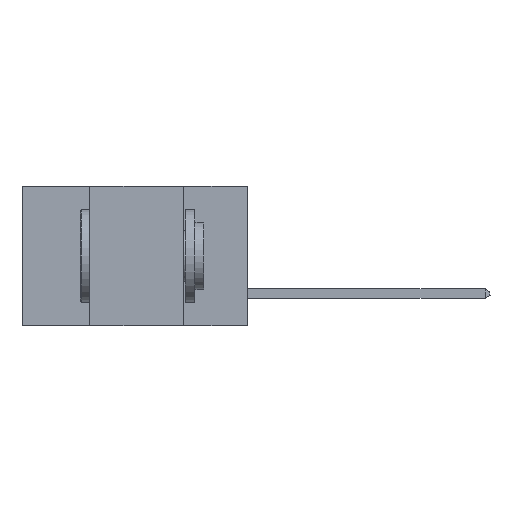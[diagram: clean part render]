
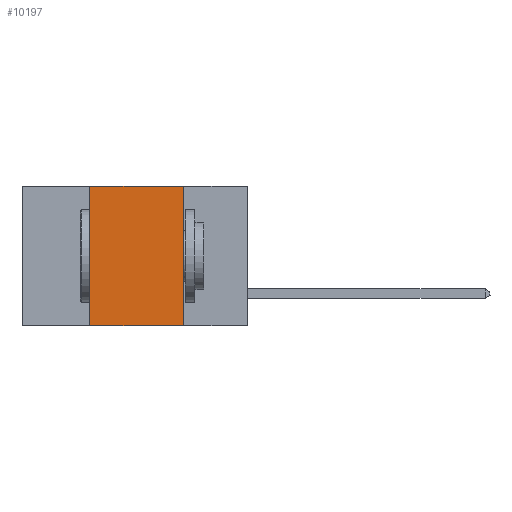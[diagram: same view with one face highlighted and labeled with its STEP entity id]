
A CAD part, left-side view. The second image highlights one B-rep face of the part: STEP entity #10197.
In plain terms, the highlighted planar face has unit normal (-1, 0, 0).
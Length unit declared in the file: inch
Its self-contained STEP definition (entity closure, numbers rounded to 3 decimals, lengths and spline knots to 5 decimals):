
#620 = ORIENTED_EDGE ( 'NONE', *, *, #3255, .F. ) ;
#631 = EDGE_CURVE ( 'NONE', #6738, #16719, #28780, .T. ) ;
#664 = VERTEX_POINT ( 'NONE', #19936 ) ;
#1987 = ORIENTED_EDGE ( 'NONE', *, *, #21892, .F. ) ;
#2713 = CARTESIAN_POINT ( 'NONE',  ( 0., 0.6, 0. ) ) ;
#2913 = PLANE ( 'NONE',  #12123 ) ;
#3255 = EDGE_CURVE ( 'NONE', #16719, #664, #14291, .T. ) ;
#3353 = VECTOR ( 'NONE', #29371, 39.37008 ) ;
#4187 = EDGE_CURVE ( 'NONE', #6738, #10161, #17978, .T. ) ;
#4322 = VECTOR ( 'NONE', #18372, 39.37008 ) ;
#4847 = CARTESIAN_POINT ( 'NONE',  ( 0., 0.6, 0. ) ) ;
#6738 = VERTEX_POINT ( 'NONE', #20843 ) ;
#7091 = VECTOR ( 'NONE', #29343, 39.37008 ) ;
#7294 = DIRECTION ( 'NONE',  ( 0., 0., -1. ) ) ;
#10161 = VERTEX_POINT ( 'NONE', #24677 ) ;
#10197 = ADVANCED_FACE ( 'NONE', ( #26248 ), #2913, .F. ) ;
#10326 = ORIENTED_EDGE ( 'NONE', *, *, #4187, .T. ) ;
#12123 = AXIS2_PLACEMENT_3D ( 'NONE', #2713, #24469, #7294 ) ;
#12476 = ORIENTED_EDGE ( 'NONE', *, *, #631, .F. ) ;
#13854 = CARTESIAN_POINT ( 'NONE',  ( 0., 0.17, 0. ) ) ;
#14291 = LINE ( 'NONE', #4847, #7091 ) ;
#14648 = CARTESIAN_POINT ( 'NONE',  ( 0., 0.42, 0. ) ) ;
#14711 = CARTESIAN_POINT ( 'NONE',  ( 0., 0.6, -0.37 ) ) ;
#16719 = VERTEX_POINT ( 'NONE', #14648 ) ;
#17325 = LINE ( 'NONE', #13854, #29846 ) ;
#17978 = LINE ( 'NONE', #14711, #4322 ) ;
#18372 = DIRECTION ( 'NONE',  ( 0., -1., 0. ) ) ;
#19936 = CARTESIAN_POINT ( 'NONE',  ( 0., 0.17, 0. ) ) ;
#20843 = CARTESIAN_POINT ( 'NONE',  ( 0., 0.42, -0.37 ) ) ;
#21318 = DIRECTION ( 'NONE',  ( 0., 0., -1. ) ) ;
#21892 = EDGE_CURVE ( 'NONE', #664, #10161, #17325, .T. ) ;
#24469 = DIRECTION ( 'NONE',  ( 1., 0., 0. ) ) ;
#24677 = CARTESIAN_POINT ( 'NONE',  ( 0., 0.17, -0.37 ) ) ;
#26248 = FACE_OUTER_BOUND ( 'NONE', #30735, .T. ) ;
#27022 = CARTESIAN_POINT ( 'NONE',  ( 0., 0.42, 0. ) ) ;
#28780 = LINE ( 'NONE', #27022, #3353 ) ;
#29343 = DIRECTION ( 'NONE',  ( 0., -1., 0. ) ) ;
#29371 = DIRECTION ( 'NONE',  ( 0., 0., 1. ) ) ;
#29846 = VECTOR ( 'NONE', #21318, 39.37008 ) ;
#30735 = EDGE_LOOP ( 'NONE', ( #1987, #620, #12476, #10326 ) ) ;
